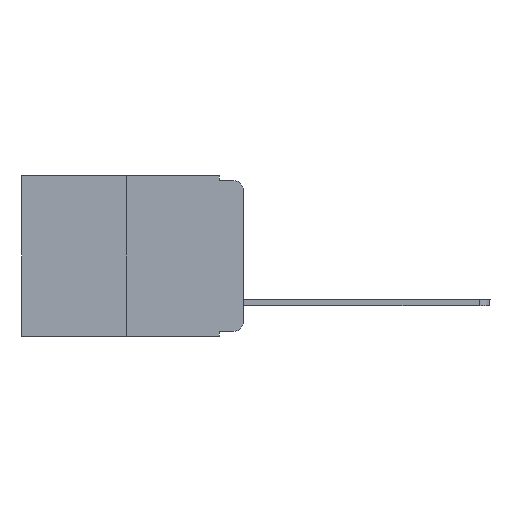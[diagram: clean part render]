
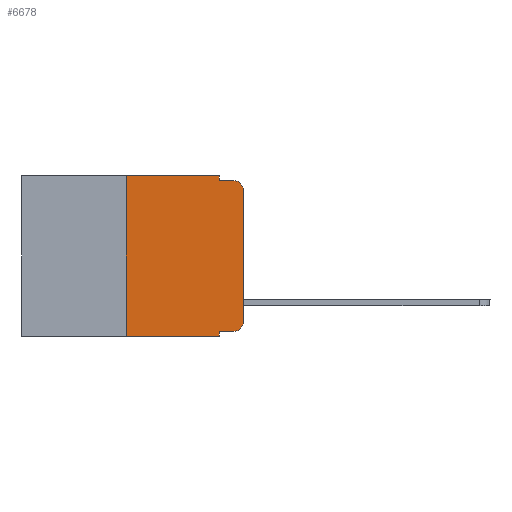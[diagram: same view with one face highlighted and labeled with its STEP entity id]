
A CAD part, left-side view. The second image highlights one B-rep face of the part: STEP entity #6678.
In plain terms, the highlighted planar face has unit normal (-1, 0, 0).
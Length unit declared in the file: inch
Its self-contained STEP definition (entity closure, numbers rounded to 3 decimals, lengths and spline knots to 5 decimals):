
#148 = CARTESIAN_POINT ( 'NONE',  ( 0., 0., 0. ) ) ;
#379 = DIRECTION ( 'NONE',  ( 0., -1., 0. ) ) ;
#626 = EDGE_CURVE ( 'NONE', #12610, #9339, #815, .T. ) ;
#734 = AXIS2_PLACEMENT_3D ( 'NONE', #9576, #1577, #8722 ) ;
#815 = CIRCLE ( 'NONE', #12664, 0.02 ) ;
#1208 = VERTEX_POINT ( 'NONE', #12898 ) ;
#1323 = ORIENTED_EDGE ( 'NONE', *, *, #3755, .F. ) ;
#1577 = DIRECTION ( 'NONE',  ( -1., 0., 0. ) ) ;
#1698 = VECTOR ( 'NONE', #12655, 39.37008 ) ;
#1724 = CARTESIAN_POINT ( 'NONE',  ( 0., 0.25, 0. ) ) ;
#1973 = VERTEX_POINT ( 'NONE', #2040 ) ;
#2018 = EDGE_CURVE ( 'NONE', #9339, #3667, #8278, .T. ) ;
#2040 = CARTESIAN_POINT ( 'NONE',  ( 0., 0.051, -0.01 ) ) ;
#2103 = CARTESIAN_POINT ( 'NONE',  ( 0., 0.02, -0.313 ) ) ;
#2214 = EDGE_CURVE ( 'NONE', #4712, #12610, #7469, .T. ) ;
#2221 = VECTOR ( 'NONE', #7340, 39.37008 ) ;
#2364 = CARTESIAN_POINT ( 'NONE',  ( 0., 0.473, -0.343 ) ) ;
#2577 = LINE ( 'NONE', #2724, #11654 ) ;
#2716 = VECTOR ( 'NONE', #3783, 39.37008 ) ;
#2724 = CARTESIAN_POINT ( 'NONE',  ( 0., 0.473, 0. ) ) ;
#2843 = LINE ( 'NONE', #5567, #1698 ) ;
#3012 = LINE ( 'NONE', #3154, #9861 ) ;
#3154 = CARTESIAN_POINT ( 'NONE',  ( 0., 0.051, 0. ) ) ;
#3186 = ORIENTED_EDGE ( 'NONE', *, *, #2214, .T. ) ;
#3604 = ORIENTED_EDGE ( 'NONE', *, *, #2018, .T. ) ;
#3629 = ORIENTED_EDGE ( 'NONE', *, *, #5913, .F. ) ;
#3667 = VERTEX_POINT ( 'NONE', #6584 ) ;
#3755 = EDGE_CURVE ( 'NONE', #4539, #8415, #2843, .T. ) ;
#3783 = DIRECTION ( 'NONE',  ( 0., 0., -1. ) ) ;
#4079 = DIRECTION ( 'NONE',  ( 0., 0., -1. ) ) ;
#4294 = DIRECTION ( 'NONE',  ( 0., -1., 0. ) ) ;
#4539 = VERTEX_POINT ( 'NONE', #7626 ) ;
#4712 = VERTEX_POINT ( 'NONE', #6348 ) ;
#4724 = CARTESIAN_POINT ( 'NONE',  ( 0., 0.051, 0. ) ) ;
#4929 = VECTOR ( 'NONE', #4294, 39.37008 ) ;
#5125 = CARTESIAN_POINT ( 'NONE',  ( 0., 0.051, -0.343 ) ) ;
#5567 = CARTESIAN_POINT ( 'NONE',  ( 0., 0.25, 0. ) ) ;
#5845 = EDGE_CURVE ( 'NONE', #4539, #11770, #11801, .T. ) ;
#5856 = ORIENTED_EDGE ( 'NONE', *, *, #5845, .T. ) ;
#5913 = EDGE_CURVE ( 'NONE', #8415, #1208, #2577, .T. ) ;
#5951 = ORIENTED_EDGE ( 'NONE', *, *, #12252, .F. ) ;
#6169 = CARTESIAN_POINT ( 'NONE',  ( 0., 0.051, -0.333 ) ) ;
#6275 = CARTESIAN_POINT ( 'NONE',  ( 0., 0.473, 0. ) ) ;
#6348 = CARTESIAN_POINT ( 'NONE',  ( 0., 0.051, -0.333 ) ) ;
#6584 = CARTESIAN_POINT ( 'NONE',  ( 0., 0., -0.03 ) ) ;
#6678 = ADVANCED_FACE ( 'NONE', ( #8290 ), #12335, .F. ) ;
#7101 = EDGE_CURVE ( 'NONE', #1208, #1973, #11005, .T. ) ;
#7311 = EDGE_CURVE ( 'NONE', #1973, #10201, #10041, .T. ) ;
#7340 = DIRECTION ( 'NONE',  ( 0., 0., 1. ) ) ;
#7469 = LINE ( 'NONE', #6169, #4929 ) ;
#7478 = EDGE_CURVE ( 'NONE', #3667, #10201, #13199, .T. ) ;
#7498 = CARTESIAN_POINT ( 'NONE',  ( 0., 0., -0.313 ) ) ;
#7626 = CARTESIAN_POINT ( 'NONE',  ( 0., 0.25, -0.343 ) ) ;
#8155 = ORIENTED_EDGE ( 'NONE', *, *, #7101, .F. ) ;
#8179 = ORIENTED_EDGE ( 'NONE', *, *, #7311, .F. ) ;
#8278 = LINE ( 'NONE', #148, #2221 ) ;
#8290 = FACE_OUTER_BOUND ( 'NONE', #9930, .T. ) ;
#8415 = VERTEX_POINT ( 'NONE', #1724 ) ;
#8494 = ORIENTED_EDGE ( 'NONE', *, *, #7478, .T. ) ;
#8722 = DIRECTION ( 'NONE',  ( 0., 0., -1. ) ) ;
#8855 = CARTESIAN_POINT ( 'NONE',  ( 0., 0.02, -0.333 ) ) ;
#8953 = VECTOR ( 'NONE', #379, 39.37008 ) ;
#9023 = AXIS2_PLACEMENT_3D ( 'NONE', #6275, #12391, #4079 ) ;
#9216 = CARTESIAN_POINT ( 'NONE',  ( 0., 0.051, -0.01 ) ) ;
#9339 = VERTEX_POINT ( 'NONE', #7498 ) ;
#9353 = DIRECTION ( 'NONE',  ( 0., 0., -1. ) ) ;
#9403 = VECTOR ( 'NONE', #11310, 39.37008 ) ;
#9576 = CARTESIAN_POINT ( 'NONE',  ( 0., 0.02, -0.03 ) ) ;
#9861 = VECTOR ( 'NONE', #9353, 39.37008 ) ;
#9930 = EDGE_LOOP ( 'NONE', ( #3604, #8494, #8179, #8155, #3629, #1323, #5856, #5951, #3186, #11742 ) ) ;
#10041 = LINE ( 'NONE', #9216, #9403 ) ;
#10201 = VERTEX_POINT ( 'NONE', #12467 ) ;
#10222 = DIRECTION ( 'NONE',  ( -1., 0., 0. ) ) ;
#10884 = DIRECTION ( 'NONE',  ( 0., -1., 0. ) ) ;
#11005 = LINE ( 'NONE', #4724, #2716 ) ;
#11310 = DIRECTION ( 'NONE',  ( 0., -1., 0. ) ) ;
#11594 = DIRECTION ( 'NONE',  ( 0., 0., -1. ) ) ;
#11654 = VECTOR ( 'NONE', #10884, 39.37008 ) ;
#11742 = ORIENTED_EDGE ( 'NONE', *, *, #626, .T. ) ;
#11770 = VERTEX_POINT ( 'NONE', #5125 ) ;
#11801 = LINE ( 'NONE', #2364, #8953 ) ;
#12252 = EDGE_CURVE ( 'NONE', #4712, #11770, #3012, .T. ) ;
#12335 = PLANE ( 'NONE',  #9023 ) ;
#12391 = DIRECTION ( 'NONE',  ( 1., 0., 0. ) ) ;
#12467 = CARTESIAN_POINT ( 'NONE',  ( 0., 0.02, -0.01 ) ) ;
#12610 = VERTEX_POINT ( 'NONE', #8855 ) ;
#12655 = DIRECTION ( 'NONE',  ( 0., 0., 1. ) ) ;
#12664 = AXIS2_PLACEMENT_3D ( 'NONE', #2103, #10222, #11594 ) ;
#12898 = CARTESIAN_POINT ( 'NONE',  ( 0., 0.051, 0. ) ) ;
#13199 = CIRCLE ( 'NONE', #734, 0.02 ) ;
